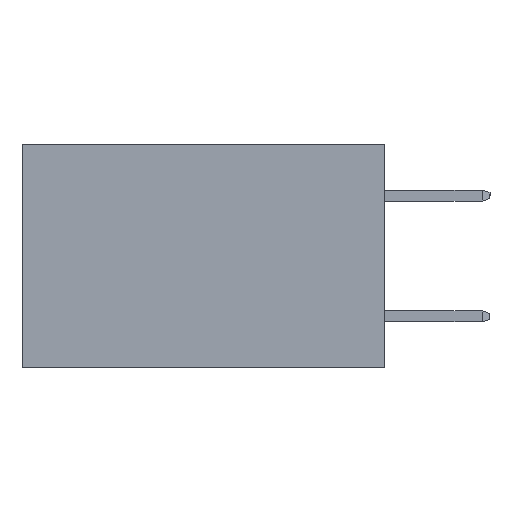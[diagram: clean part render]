
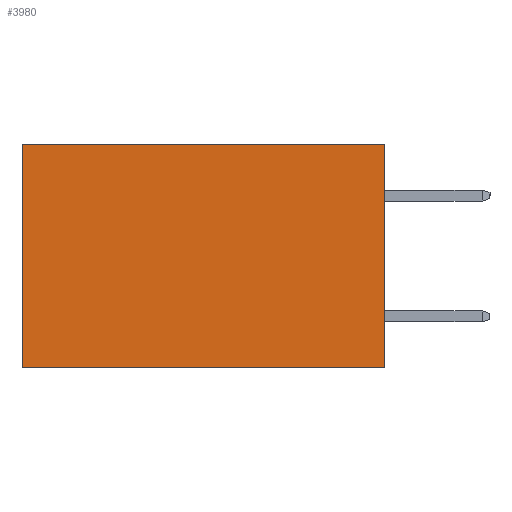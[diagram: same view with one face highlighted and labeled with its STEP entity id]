
A CAD part, left-side view. The second image highlights one B-rep face of the part: STEP entity #3980.
In plain terms, the highlighted planar face has unit normal (-1, 0, 0).
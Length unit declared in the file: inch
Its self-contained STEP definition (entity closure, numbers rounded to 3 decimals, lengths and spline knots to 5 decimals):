
#397 = DIRECTION ( 'NONE',  ( 0., 0., -1. ) ) ;
#564 = DIRECTION ( 'NONE',  ( 1., 0., 0. ) ) ;
#731 = CARTESIAN_POINT ( 'NONE',  ( 0.2615, 0.6, -0.37 ) ) ;
#1062 = EDGE_CURVE ( 'NONE', #7617, #8610, #7159, .T. ) ;
#1281 = AXIS2_PLACEMENT_3D ( 'NONE', #8643, #564, #5601 ) ;
#1372 = ORIENTED_EDGE ( 'NONE', *, *, #8351, .F. ) ;
#1523 = LINE ( 'NONE', #2121, #3091 ) ;
#1681 = LINE ( 'NONE', #4533, #4354 ) ;
#1910 = CARTESIAN_POINT ( 'NONE',  ( 0.2615, 0., 0. ) ) ;
#1967 = CARTESIAN_POINT ( 'NONE',  ( 0.2615, 0.6, -0.37 ) ) ;
#2067 = DIRECTION ( 'NONE',  ( 0., 1., 0. ) ) ;
#2121 = CARTESIAN_POINT ( 'NONE',  ( 0.2615, 0., -0.37 ) ) ;
#2137 = CARTESIAN_POINT ( 'NONE',  ( 0.2615, 0.6, 0. ) ) ;
#3091 = VECTOR ( 'NONE', #2067, 39.37008 ) ;
#3450 = CARTESIAN_POINT ( 'NONE',  ( 0.2615, 0., 0. ) ) ;
#3980 = ADVANCED_FACE ( 'NONE', ( #9285 ), #9196, .F. ) ;
#3984 = VECTOR ( 'NONE', #7907, 39.37008 ) ;
#4207 = DIRECTION ( 'NONE',  ( 0., 1., 0. ) ) ;
#4354 = VECTOR ( 'NONE', #397, 39.37008 ) ;
#4533 = CARTESIAN_POINT ( 'NONE',  ( 0.2615, 0., -0.37 ) ) ;
#4707 = ORIENTED_EDGE ( 'NONE', *, *, #1062, .T. ) ;
#5198 = LINE ( 'NONE', #731, #3984 ) ;
#5271 = VERTEX_POINT ( 'NONE', #1967 ) ;
#5397 = EDGE_CURVE ( 'NONE', #7253, #5271, #1523, .T. ) ;
#5404 = VECTOR ( 'NONE', #4207, 39.37008 ) ;
#5492 = ORIENTED_EDGE ( 'NONE', *, *, #5397, .F. ) ;
#5601 = DIRECTION ( 'NONE',  ( 0., 0., -1. ) ) ;
#6395 = ORIENTED_EDGE ( 'NONE', *, *, #8555, .T. ) ;
#6523 = CARTESIAN_POINT ( 'NONE',  ( 0.2615, 0., -0.37 ) ) ;
#7159 = LINE ( 'NONE', #3450, #5404 ) ;
#7253 = VERTEX_POINT ( 'NONE', #6523 ) ;
#7617 = VERTEX_POINT ( 'NONE', #1910 ) ;
#7875 = EDGE_LOOP ( 'NONE', ( #6395, #5492, #1372, #4707 ) ) ;
#7907 = DIRECTION ( 'NONE',  ( 0., 0., -1. ) ) ;
#8351 = EDGE_CURVE ( 'NONE', #7617, #7253, #1681, .T. ) ;
#8555 = EDGE_CURVE ( 'NONE', #8610, #5271, #5198, .T. ) ;
#8610 = VERTEX_POINT ( 'NONE', #2137 ) ;
#8643 = CARTESIAN_POINT ( 'NONE',  ( 0.2615, 0., -0.37 ) ) ;
#9196 = PLANE ( 'NONE',  #1281 ) ;
#9285 = FACE_OUTER_BOUND ( 'NONE', #7875, .T. ) ;
